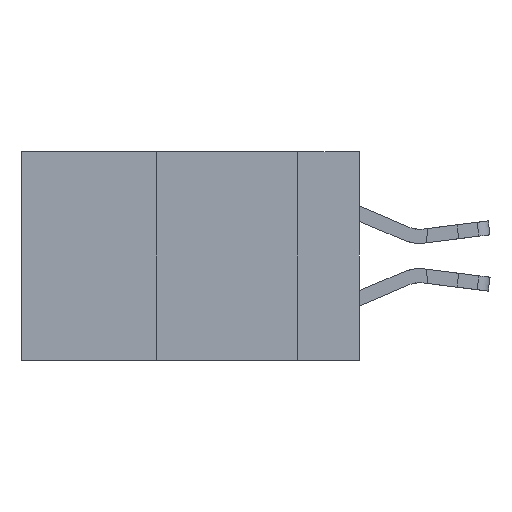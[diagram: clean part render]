
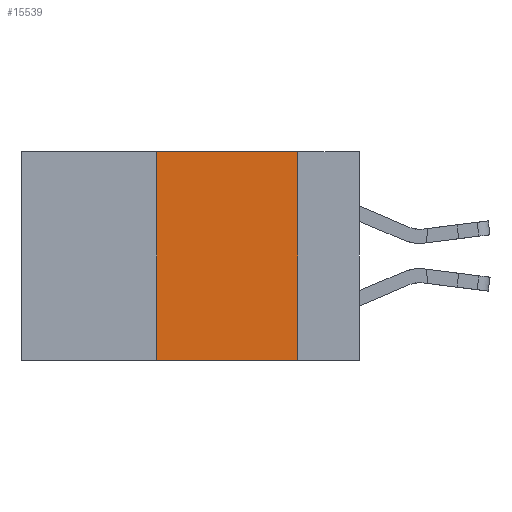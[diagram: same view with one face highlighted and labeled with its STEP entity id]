
A CAD part, left-side view. The second image highlights one B-rep face of the part: STEP entity #15539.
In plain terms, the highlighted planar face has unit normal (-1, 0, 0).
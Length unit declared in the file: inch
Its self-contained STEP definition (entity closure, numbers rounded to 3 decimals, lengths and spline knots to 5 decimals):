
#53 = VERTEX_POINT ( 'NONE', #10396 ) ;
#87 = LINE ( 'NONE', #9483, #5496 ) ;
#2177 = FACE_OUTER_BOUND ( 'NONE', #4664, .T. ) ;
#2541 = ORIENTED_EDGE ( 'NONE', *, *, #3318, .F. ) ;
#3318 = EDGE_CURVE ( 'NONE', #6225, #13609, #9415, .T. ) ;
#4479 = DIRECTION ( 'NONE',  ( 0., 0., -1. ) ) ;
#4664 = EDGE_LOOP ( 'NONE', ( #6948, #2541, #14346, #10290 ) ) ;
#5496 = VECTOR ( 'NONE', #13149, 39.37008 ) ;
#5648 = DIRECTION ( 'NONE',  ( 1., 0., 0. ) ) ;
#5676 = CARTESIAN_POINT ( 'NONE',  ( 0., 0.11, -0.37 ) ) ;
#5759 = AXIS2_PLACEMENT_3D ( 'NONE', #7991, #5648, #4479 ) ;
#5867 = DIRECTION ( 'NONE',  ( 0., 0., -1. ) ) ;
#6225 = VERTEX_POINT ( 'NONE', #13656 ) ;
#6948 = ORIENTED_EDGE ( 'NONE', *, *, #7024, .F. ) ;
#6992 = CARTESIAN_POINT ( 'NONE',  ( 0., 0.11, 0. ) ) ;
#7024 = EDGE_CURVE ( 'NONE', #13609, #8049, #12499, .T. ) ;
#7991 = CARTESIAN_POINT ( 'NONE',  ( 0., 0.6, 0. ) ) ;
#8049 = VERTEX_POINT ( 'NONE', #5676 ) ;
#8261 = DIRECTION ( 'NONE',  ( 0., -1., 0. ) ) ;
#8822 = VECTOR ( 'NONE', #8261, 39.37008 ) ;
#9221 = EDGE_CURVE ( 'NONE', #53, #8049, #15306, .T. ) ;
#9415 = LINE ( 'NONE', #14308, #8822 ) ;
#9483 = CARTESIAN_POINT ( 'NONE',  ( 0., 0.36, 0. ) ) ;
#10006 = VECTOR ( 'NONE', #14749, 39.37008 ) ;
#10290 = ORIENTED_EDGE ( 'NONE', *, *, #9221, .T. ) ;
#10396 = CARTESIAN_POINT ( 'NONE',  ( 0., 0.36, -0.37 ) ) ;
#11109 = CARTESIAN_POINT ( 'NONE',  ( 0., 0.6, -0.37 ) ) ;
#11830 = EDGE_CURVE ( 'NONE', #53, #6225, #87, .T. ) ;
#12499 = LINE ( 'NONE', #6992, #15161 ) ;
#13149 = DIRECTION ( 'NONE',  ( 0., 0., 1. ) ) ;
#13609 = VERTEX_POINT ( 'NONE', #15056 ) ;
#13656 = CARTESIAN_POINT ( 'NONE',  ( 0., 0.36, 0. ) ) ;
#14034 = PLANE ( 'NONE',  #5759 ) ;
#14308 = CARTESIAN_POINT ( 'NONE',  ( 0., 0.6, 0. ) ) ;
#14346 = ORIENTED_EDGE ( 'NONE', *, *, #11830, .F. ) ;
#14749 = DIRECTION ( 'NONE',  ( 0., -1., 0. ) ) ;
#15056 = CARTESIAN_POINT ( 'NONE',  ( 0., 0.11, 0. ) ) ;
#15161 = VECTOR ( 'NONE', #5867, 39.37008 ) ;
#15306 = LINE ( 'NONE', #11109, #10006 ) ;
#15539 = ADVANCED_FACE ( 'NONE', ( #2177 ), #14034, .F. ) ;
